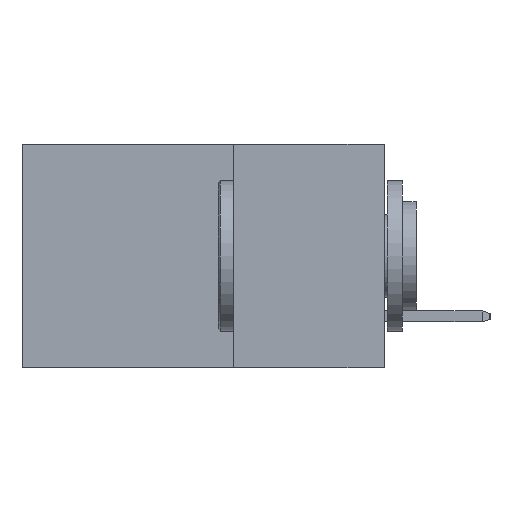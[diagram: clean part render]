
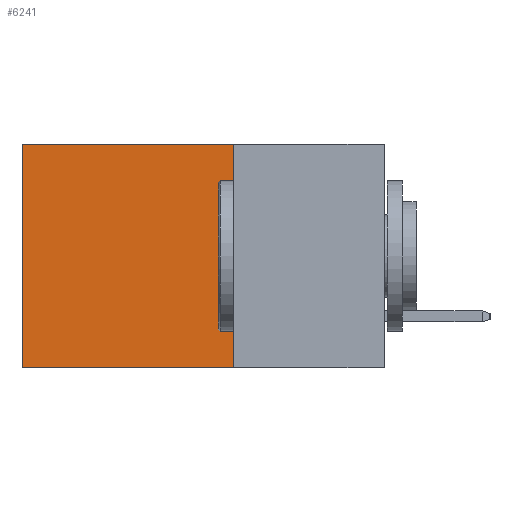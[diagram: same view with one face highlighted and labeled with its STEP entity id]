
A CAD part, left-side view. The second image highlights one B-rep face of the part: STEP entity #6241.
In plain terms, the highlighted planar face has unit normal (-1, 0, 0).
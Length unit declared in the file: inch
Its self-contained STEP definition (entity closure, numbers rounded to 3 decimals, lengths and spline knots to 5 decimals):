
#216 = LINE ( 'NONE', #7250, #4287 ) ;
#217 = DIRECTION ( 'NONE',  ( 1., 0., 0. ) ) ;
#314 = DIRECTION ( 'NONE',  ( 0., 1., 0. ) ) ;
#936 = PLANE ( 'NONE',  #5328 ) ;
#993 = VECTOR ( 'NONE', #4493, 39.37008 ) ;
#1733 = CARTESIAN_POINT ( 'NONE',  ( 0.2615, 0.25, 0. ) ) ;
#2308 = CARTESIAN_POINT ( 'NONE',  ( 0.2615, 0.25, -0.37 ) ) ;
#2447 = ORIENTED_EDGE ( 'NONE', *, *, #8651, .T. ) ;
#2542 = CARTESIAN_POINT ( 'NONE',  ( 0.2615, 0.25, -0.37 ) ) ;
#2672 = VECTOR ( 'NONE', #5530, 39.37008 ) ;
#2957 = CARTESIAN_POINT ( 'NONE',  ( 0.2615, 0.6, 0. ) ) ;
#3276 = VERTEX_POINT ( 'NONE', #2308 ) ;
#3286 = VECTOR ( 'NONE', #314, 39.37008 ) ;
#4287 = VECTOR ( 'NONE', #5071, 39.37008 ) ;
#4453 = CARTESIAN_POINT ( 'NONE',  ( 0.2615, 0.6, -0.37 ) ) ;
#4493 = DIRECTION ( 'NONE',  ( 0., 0., -1. ) ) ;
#4919 = EDGE_CURVE ( 'NONE', #7685, #7926, #6767, .T. ) ;
#5071 = DIRECTION ( 'NONE',  ( 0., 0., -1. ) ) ;
#5304 = EDGE_LOOP ( 'NONE', ( #9263, #8054, #5374, #2447 ) ) ;
#5328 = AXIS2_PLACEMENT_3D ( 'NONE', #2542, #217, #5545 ) ;
#5374 = ORIENTED_EDGE ( 'NONE', *, *, #8928, .F. ) ;
#5530 = DIRECTION ( 'NONE',  ( 0., 1., 0. ) ) ;
#5545 = DIRECTION ( 'NONE',  ( 0., 0., -1. ) ) ;
#6241 = ADVANCED_FACE ( 'NONE', ( #6289 ), #936, .F. ) ;
#6289 = FACE_OUTER_BOUND ( 'NONE', #5304, .T. ) ;
#6590 = LINE ( 'NONE', #1733, #2672 ) ;
#6643 = VERTEX_POINT ( 'NONE', #8848 ) ;
#6767 = LINE ( 'NONE', #4453, #993 ) ;
#6954 = CARTESIAN_POINT ( 'NONE',  ( 0.2615, 0.6, -0.37 ) ) ;
#7250 = CARTESIAN_POINT ( 'NONE',  ( 0.2615, 0.25, -0.37 ) ) ;
#7460 = EDGE_CURVE ( 'NONE', #3276, #7926, #9067, .T. ) ;
#7685 = VERTEX_POINT ( 'NONE', #2957 ) ;
#7926 = VERTEX_POINT ( 'NONE', #6954 ) ;
#8054 = ORIENTED_EDGE ( 'NONE', *, *, #7460, .F. ) ;
#8651 = EDGE_CURVE ( 'NONE', #6643, #7685, #6590, .T. ) ;
#8848 = CARTESIAN_POINT ( 'NONE',  ( 0.2615, 0.25, 0. ) ) ;
#8928 = EDGE_CURVE ( 'NONE', #6643, #3276, #216, .T. ) ;
#9067 = LINE ( 'NONE', #9195, #3286 ) ;
#9195 = CARTESIAN_POINT ( 'NONE',  ( 0.2615, 0.25, -0.37 ) ) ;
#9263 = ORIENTED_EDGE ( 'NONE', *, *, #4919, .T. ) ;
